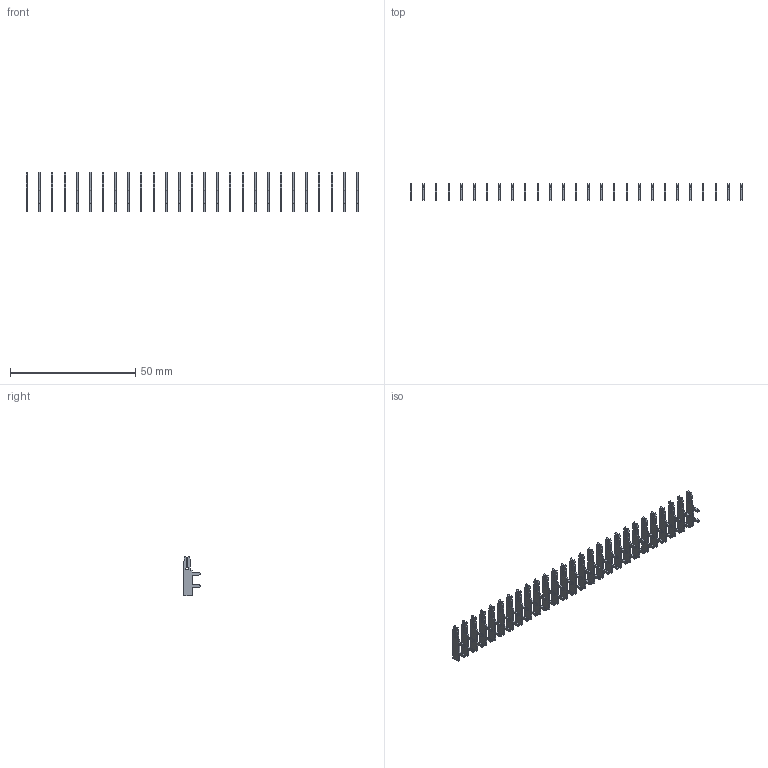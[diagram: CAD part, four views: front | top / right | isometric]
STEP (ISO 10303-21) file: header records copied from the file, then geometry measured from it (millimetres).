
FILE_DESCRIPTION (( 'STEP AP203' ), '1' );
FILE_NAME ('105-027-202-200.STEP', '2020-04-07T23:17:06', ( '' ), ( '' ), 'SwSTEP 2.0', 'SolidWorks 2016', '' );
FILE_SCHEMA (( 'CONFIG_CONTROL_DESIGN' ));
Length unit declared in the file: inch
Products named in the file (2): 105-027-202-200; 100-290-001_100-290-202
Assembly tree (27 placements, depth 2):
  105-027-202-200
    100-290-001_100-290-202  x27
Bounding box: 132.68 x 6.53 x 15.88 mm (x, y, z)
Volume: 857.8 mm3; surface area: 3815.1 mm2
Topology: 27 solids, 27 shells, 810 faces, 2268 edges, 1512 vertices
Faces by surface type: plane 621, cylinder 189
Entity records: 1994 total; most frequent: DIRECTION 214, CARTESIAN_POINT 212, ORIENTED_EDGE 168, EDGE_CURVE 84, AXIS2_PLACEMENT_3D 74, LINE 66, VECTOR 66, COORDINATED_UNIVERSAL_TIME_OFFSET 64
